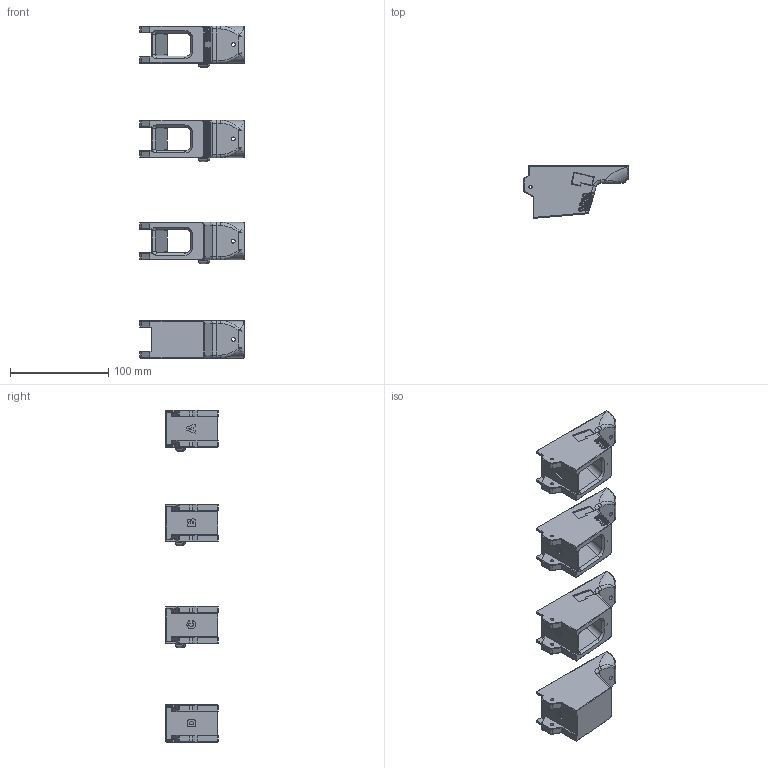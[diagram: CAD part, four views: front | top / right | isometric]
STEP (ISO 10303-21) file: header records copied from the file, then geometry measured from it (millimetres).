
FILE_DESCRIPTION(/* description */ (''),/* implementation_level */ '2;1');
FILE_NAME(/* name */ 'Quick Print Magwells G17.G19.stp',/* time_stamp */ '2020-10-20T12:03:52+03:00',/* author */ (''),/* organization */ (''),/* preprocessor_version */ 'ST-DEVELOPER v15.2',/* originating_system */ 'Autodesk Translator Framework v2.0.0.5431',/* authorisation */ '');
FILE_SCHEMA (('AUTOMOTIVE_DESIGN { 1 0 10303 214 3 1 1 }'));
Length unit declared in the file: centimetre
Products named in the file (1): MOD9 QUICK PRINT MAGWELL
Bounding box: 106.51 x 53.17 x 338 mm (x, y, z)
Volume: 408588.1 mm3; surface area: 101834.4 mm2
Topology: 7 solids, 7 shells, 1918 faces, 4688 edges, 2749 vertices
Faces by surface type: cylinder 640, bspline 578, plane 554, sphere 68, torus 48, cone 30
Full cylindrical faces by diameter (mm): 1.5 x6, 3.4 x8, 4 x8
Entity records: 66558 total; most frequent: CARTESIAN_POINT 24514, ORIENTED_EDGE 9232, DIRECTION 7844, EDGE_CURVE 4616, AXIS2_PLACEMENT_3D 2750, VERTEX_POINT 2746, LINE 2344, VECTOR 2344
